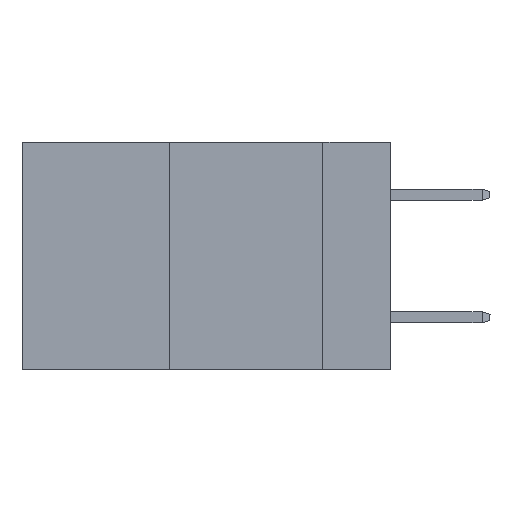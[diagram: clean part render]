
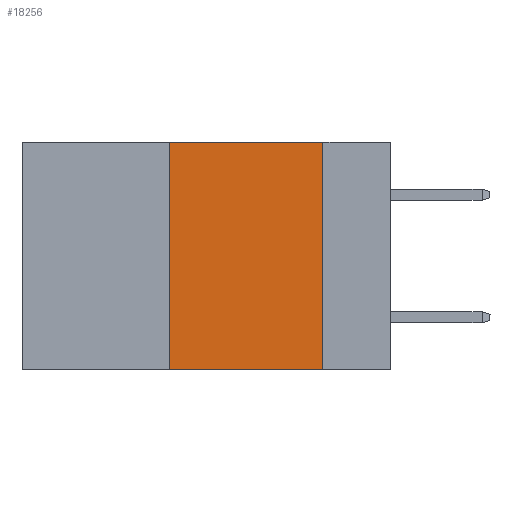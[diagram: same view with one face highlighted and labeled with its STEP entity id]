
A CAD part, left-side view. The second image highlights one B-rep face of the part: STEP entity #18256.
In plain terms, the highlighted planar face has unit normal (-1, 0, 0).
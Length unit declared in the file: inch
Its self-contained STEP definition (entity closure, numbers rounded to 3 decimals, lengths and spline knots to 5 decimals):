
#247 = CARTESIAN_POINT ( 'NONE',  ( 0., 0.36, 0. ) ) ;
#918 = EDGE_CURVE ( 'NONE', #32050, #18115, #36579, .T. ) ;
#6544 = LINE ( 'NONE', #18751, #42267 ) ;
#8426 = VECTOR ( 'NONE', #26761, 39.37008 ) ;
#12357 = CARTESIAN_POINT ( 'NONE',  ( 0., 0.36, -0.37 ) ) ;
#13140 = ORIENTED_EDGE ( 'NONE', *, *, #39872, .F. ) ;
#13995 = CARTESIAN_POINT ( 'NONE',  ( 0., 0.6, 0. ) ) ;
#15709 = VERTEX_POINT ( 'NONE', #23925 ) ;
#16442 = CARTESIAN_POINT ( 'NONE',  ( 0., 0.6, 0. ) ) ;
#16873 = CARTESIAN_POINT ( 'NONE',  ( 0., 0.11, 0. ) ) ;
#16909 = ORIENTED_EDGE ( 'NONE', *, *, #17284, .F. ) ;
#17284 = EDGE_CURVE ( 'NONE', #35546, #32050, #6544, .T. ) ;
#17625 = DIRECTION ( 'NONE',  ( 1., 0., 0. ) ) ;
#18115 = VERTEX_POINT ( 'NONE', #16873 ) ;
#18256 = ADVANCED_FACE ( 'NONE', ( #37285 ), #20965, .F. ) ;
#18751 = CARTESIAN_POINT ( 'NONE',  ( 0., 0.36, 0. ) ) ;
#18806 = CARTESIAN_POINT ( 'NONE',  ( 0., 0.11, 0. ) ) ;
#20965 = PLANE ( 'NONE',  #26598 ) ;
#21553 = LINE ( 'NONE', #18806, #24256 ) ;
#23925 = CARTESIAN_POINT ( 'NONE',  ( 0., 0.11, -0.37 ) ) ;
#24256 = VECTOR ( 'NONE', #32557, 39.37008 ) ;
#24592 = DIRECTION ( 'NONE',  ( 0., 0., -1. ) ) ;
#26598 = AXIS2_PLACEMENT_3D ( 'NONE', #13995, #17625, #24592 ) ;
#26761 = DIRECTION ( 'NONE',  ( 0., -1., 0. ) ) ;
#27137 = ORIENTED_EDGE ( 'NONE', *, *, #918, .F. ) ;
#29590 = LINE ( 'NONE', #39849, #34433 ) ;
#29615 = EDGE_CURVE ( 'NONE', #35546, #15709, #29590, .T. ) ;
#32050 = VERTEX_POINT ( 'NONE', #247 ) ;
#32557 = DIRECTION ( 'NONE',  ( 0., 0., -1. ) ) ;
#33180 = DIRECTION ( 'NONE',  ( 0., -1., 0. ) ) ;
#34399 = EDGE_LOOP ( 'NONE', ( #13140, #27137, #16909, #41172 ) ) ;
#34433 = VECTOR ( 'NONE', #33180, 39.37008 ) ;
#35546 = VERTEX_POINT ( 'NONE', #12357 ) ;
#36579 = LINE ( 'NONE', #16442, #8426 ) ;
#37285 = FACE_OUTER_BOUND ( 'NONE', #34399, .T. ) ;
#39606 = DIRECTION ( 'NONE',  ( 0., 0., 1. ) ) ;
#39849 = CARTESIAN_POINT ( 'NONE',  ( 0., 0.6, -0.37 ) ) ;
#39872 = EDGE_CURVE ( 'NONE', #18115, #15709, #21553, .T. ) ;
#41172 = ORIENTED_EDGE ( 'NONE', *, *, #29615, .T. ) ;
#42267 = VECTOR ( 'NONE', #39606, 39.37008 ) ;
